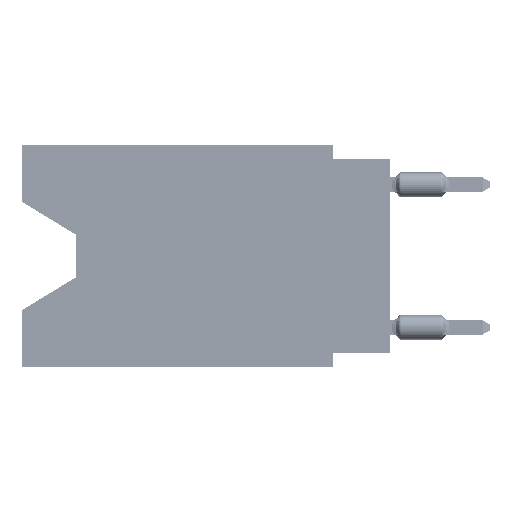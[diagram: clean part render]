
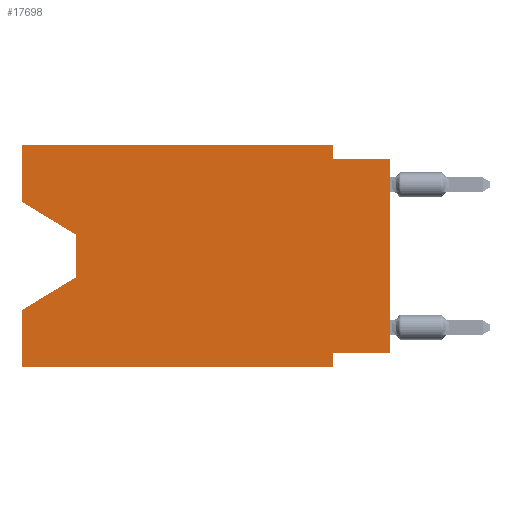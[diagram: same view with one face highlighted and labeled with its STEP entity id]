
A CAD part, left-side view. The second image highlights one B-rep face of the part: STEP entity #17698.
In plain terms, the highlighted planar face has unit normal (-1, 0, 0).
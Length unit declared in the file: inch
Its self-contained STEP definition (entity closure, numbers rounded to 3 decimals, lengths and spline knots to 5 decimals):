
#438 = CARTESIAN_POINT ( 'NONE',  ( 0., 0., 0. ) ) ;
#696 = VERTEX_POINT ( 'NONE', #23251 ) ;
#1007 = CARTESIAN_POINT ( 'NONE',  ( 0., 0., -0.365 ) ) ;
#1350 = VERTEX_POINT ( 'NONE', #5699 ) ;
#2084 = EDGE_CURVE ( 'NONE', #43795, #34046, #24981, .T. ) ;
#2360 = CARTESIAN_POINT ( 'NONE',  ( 0., 0.55, -0.158 ) ) ;
#3252 = VECTOR ( 'NONE', #40586, 39.37008 ) ;
#5374 = EDGE_LOOP ( 'NONE', ( #57560, #9792, #28033, #40964, #33385, #62879, #11732, #28275, #21604, #34452, #56652, #25016 ) ) ;
#5699 = CARTESIAN_POINT ( 'NONE',  ( 0., 0., -0.025 ) ) ;
#5950 = DIRECTION ( 'NONE',  ( 0., 1., 0. ) ) ;
#7895 = LINE ( 'NONE', #56926, #24359 ) ;
#8294 = DIRECTION ( 'NONE',  ( 0., 0., -1. ) ) ;
#8953 = LINE ( 'NONE', #58967, #49090 ) ;
#9792 = ORIENTED_EDGE ( 'NONE', *, *, #54021, .T. ) ;
#9894 = CARTESIAN_POINT ( 'NONE',  ( 0., 0.645, 0. ) ) ;
#10588 = CARTESIAN_POINT ( 'NONE',  ( 0., 0.55, -0.232 ) ) ;
#10666 = VECTOR ( 'NONE', #5950, 39.37008 ) ;
#11562 = LINE ( 'NONE', #57306, #46797 ) ;
#11732 = ORIENTED_EDGE ( 'NONE', *, *, #46532, .F. ) ;
#11936 = LINE ( 'NONE', #438, #3252 ) ;
#12846 = CARTESIAN_POINT ( 'NONE',  ( 0., 0.645, 0. ) ) ;
#12872 = EDGE_CURVE ( 'NONE', #49146, #34013, #51071, .T. ) ;
#15455 = LINE ( 'NONE', #60845, #60275 ) ;
#15528 = DIRECTION ( 'NONE',  ( 0., 0.855, -0.519 ) ) ;
#16301 = VERTEX_POINT ( 'NONE', #35928 ) ;
#16500 = DIRECTION ( 'NONE',  ( 0., -1., 0. ) ) ;
#17470 = CARTESIAN_POINT ( 'NONE',  ( 0., 0.645, 0. ) ) ;
#17698 = ADVANCED_FACE ( 'NONE', ( #52032 ), #27040, .F. ) ;
#18931 = VECTOR ( 'NONE', #15528, 39.37008 ) ;
#20206 = CARTESIAN_POINT ( 'NONE',  ( 0., 0.1, -0.39 ) ) ;
#21049 = CARTESIAN_POINT ( 'NONE',  ( 0., 0.645, -0.39 ) ) ;
#21604 = ORIENTED_EDGE ( 'NONE', *, *, #46612, .F. ) ;
#21795 = LINE ( 'NONE', #2360, #38767 ) ;
#23251 = CARTESIAN_POINT ( 'NONE',  ( 0., 0.1, -0.365 ) ) ;
#23805 = EDGE_CURVE ( 'NONE', #34046, #16301, #11562, .T. ) ;
#24359 = VECTOR ( 'NONE', #41482, 39.37008 ) ;
#24464 = VECTOR ( 'NONE', #44776, 39.37008 ) ;
#24689 = CARTESIAN_POINT ( 'NONE',  ( 0., 0.55, -0.232 ) ) ;
#24981 = LINE ( 'NONE', #45690, #42638 ) ;
#25016 = ORIENTED_EDGE ( 'NONE', *, *, #2084, .F. ) ;
#26240 = VERTEX_POINT ( 'NONE', #28663 ) ;
#26749 = DIRECTION ( 'NONE',  ( 0., 0., -1. ) ) ;
#27040 = PLANE ( 'NONE',  #55859 ) ;
#28022 = DIRECTION ( 'NONE',  ( 0., 0., -1. ) ) ;
#28033 = ORIENTED_EDGE ( 'NONE', *, *, #12872, .T. ) ;
#28275 = ORIENTED_EDGE ( 'NONE', *, *, #56336, .T. ) ;
#28663 = CARTESIAN_POINT ( 'NONE',  ( 0., 0.55, -0.158 ) ) ;
#30217 = VERTEX_POINT ( 'NONE', #46175 ) ;
#30974 = LINE ( 'NONE', #9894, #24464 ) ;
#31907 = EDGE_CURVE ( 'NONE', #43795, #26240, #48778, .T. ) ;
#33385 = ORIENTED_EDGE ( 'NONE', *, *, #40188, .T. ) ;
#34013 = VERTEX_POINT ( 'NONE', #37841 ) ;
#34046 = VERTEX_POINT ( 'NONE', #17470 ) ;
#34452 = ORIENTED_EDGE ( 'NONE', *, *, #61239, .F. ) ;
#34736 = VERTEX_POINT ( 'NONE', #37042 ) ;
#34744 = VERTEX_POINT ( 'NONE', #56462 ) ;
#35862 = DIRECTION ( 'NONE',  ( 0., 0., -1. ) ) ;
#35928 = CARTESIAN_POINT ( 'NONE',  ( 0., 0.1, 0. ) ) ;
#37042 = CARTESIAN_POINT ( 'NONE',  ( 0., 0.645, -0.39 ) ) ;
#37841 = CARTESIAN_POINT ( 'NONE',  ( 0., 0.645, -0.28975 ) ) ;
#38199 = EDGE_CURVE ( 'NONE', #696, #47269, #8953, .T. ) ;
#38767 = VECTOR ( 'NONE', #26749, 39.37008 ) ;
#40188 = EDGE_CURVE ( 'NONE', #34736, #47269, #57205, .T. ) ;
#40434 = DIRECTION ( 'NONE',  ( 0., 0., 1. ) ) ;
#40586 = DIRECTION ( 'NONE',  ( 0., 0., 1. ) ) ;
#40825 = LINE ( 'NONE', #1007, #10666 ) ;
#40964 = ORIENTED_EDGE ( 'NONE', *, *, #60272, .F. ) ;
#41482 = DIRECTION ( 'NONE',  ( 0., -1., 0. ) ) ;
#42638 = VECTOR ( 'NONE', #40434, 39.37008 ) ;
#43795 = VERTEX_POINT ( 'NONE', #64387 ) ;
#43836 = CARTESIAN_POINT ( 'NONE',  ( 0., 0.645, -0.10025 ) ) ;
#44776 = DIRECTION ( 'NONE',  ( 0., 0., 1. ) ) ;
#45050 = VECTOR ( 'NONE', #61819, 39.37008 ) ;
#45690 = CARTESIAN_POINT ( 'NONE',  ( 0., 0.645, 0. ) ) ;
#46175 = CARTESIAN_POINT ( 'NONE',  ( 0., 0.1, -0.025 ) ) ;
#46532 = EDGE_CURVE ( 'NONE', #34744, #696, #40825, .T. ) ;
#46612 = EDGE_CURVE ( 'NONE', #30217, #1350, #7895, .T. ) ;
#46797 = VECTOR ( 'NONE', #16500, 39.37008 ) ;
#47085 = DIRECTION ( 'NONE',  ( 1., 0., 0. ) ) ;
#47269 = VERTEX_POINT ( 'NONE', #20206 ) ;
#48778 = LINE ( 'NONE', #43836, #56188 ) ;
#49090 = VECTOR ( 'NONE', #8294, 39.37008 ) ;
#49146 = VERTEX_POINT ( 'NONE', #24689 ) ;
#51071 = LINE ( 'NONE', #10588, #18931 ) ;
#52032 = FACE_OUTER_BOUND ( 'NONE', #5374, .T. ) ;
#54021 = EDGE_CURVE ( 'NONE', #26240, #49146, #21795, .T. ) ;
#55859 = AXIS2_PLACEMENT_3D ( 'NONE', #12846, #47085, #28022 ) ;
#56188 = VECTOR ( 'NONE', #63905, 39.37008 ) ;
#56336 = EDGE_CURVE ( 'NONE', #34744, #1350, #11936, .T. ) ;
#56462 = CARTESIAN_POINT ( 'NONE',  ( 0., 0., -0.365 ) ) ;
#56652 = ORIENTED_EDGE ( 'NONE', *, *, #23805, .F. ) ;
#56926 = CARTESIAN_POINT ( 'NONE',  ( 0., 0., -0.025 ) ) ;
#57205 = LINE ( 'NONE', #21049, #45050 ) ;
#57306 = CARTESIAN_POINT ( 'NONE',  ( 0., 0.645, 0. ) ) ;
#57560 = ORIENTED_EDGE ( 'NONE', *, *, #31907, .T. ) ;
#58967 = CARTESIAN_POINT ( 'NONE',  ( 0., 0.1, -0.39 ) ) ;
#60272 = EDGE_CURVE ( 'NONE', #34736, #34013, #30974, .T. ) ;
#60275 = VECTOR ( 'NONE', #35862, 39.37008 ) ;
#60845 = CARTESIAN_POINT ( 'NONE',  ( 0., 0.1, 0. ) ) ;
#61239 = EDGE_CURVE ( 'NONE', #16301, #30217, #15455, .T. ) ;
#61819 = DIRECTION ( 'NONE',  ( 0., -1., 0. ) ) ;
#62879 = ORIENTED_EDGE ( 'NONE', *, *, #38199, .F. ) ;
#63905 = DIRECTION ( 'NONE',  ( 0., -0.855, -0.519 ) ) ;
#64387 = CARTESIAN_POINT ( 'NONE',  ( 0., 0.645, -0.10025 ) ) ;
